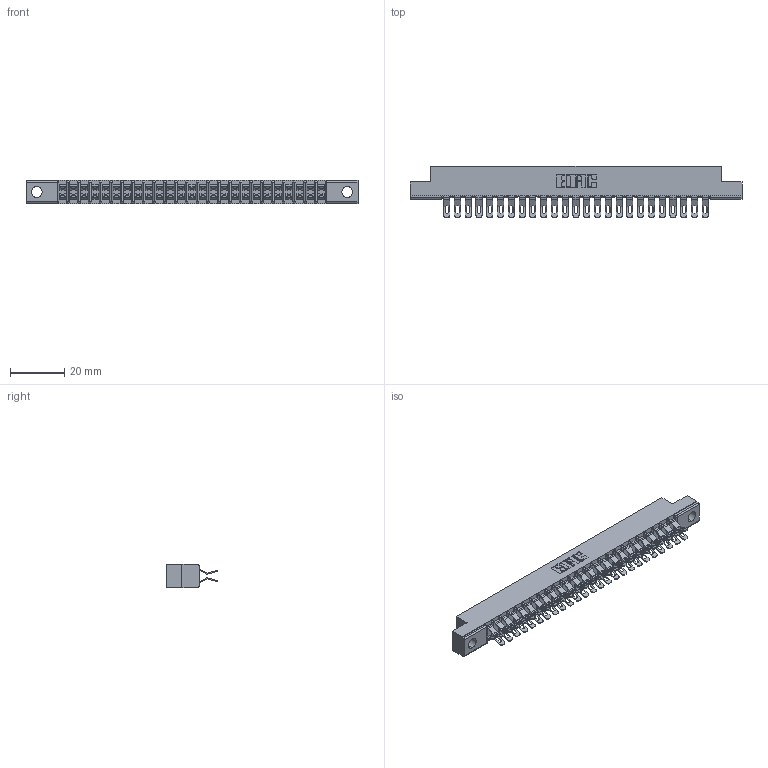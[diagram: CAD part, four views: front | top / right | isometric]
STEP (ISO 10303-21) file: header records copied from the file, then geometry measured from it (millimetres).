
FILE_DESCRIPTION (( 'STEP AP203' ), '1' );
FILE_NAME ('357-050-455-204.STEP', '2020-10-04T05:49:44', ( '' ), ( '' ), 'SwSTEP 2.0', 'SolidWorks 2020', '' );
FILE_SCHEMA (( 'CONFIG_CONTROL_DESIGN' ));
Length unit declared in the file: inch
Products named in the file (3): 307-290-001_555; 307 Part_.156 Dia Mounting Holes; 357-050-455-204
Assembly tree (51 placements, depth 2):
  357-050-455-204
    307 Part_.156 Dia Mounting Holes
    307-290-001_555  x50
Bounding box: 122.07 x 18.75 x 8.71 mm (x, y, z)
Volume: 8027.5 mm3; surface area: 15046.3 mm2
Topology: 51 solids, 51 shells, 3208 faces, 9409 edges, 6134 vertices
Faces by surface type: plane 1784, cylinder 1372, sphere 52
Entity records: 25283 total; most frequent: CARTESIAN_POINT 4151, ORIENTED_EDGE 4112, DIRECTION 4072, EDGE_CURVE 2056, LINE 1566, VECTOR 1566, VERTEX_POINT 1332, AXIS2_PLACEMENT_3D 1253
